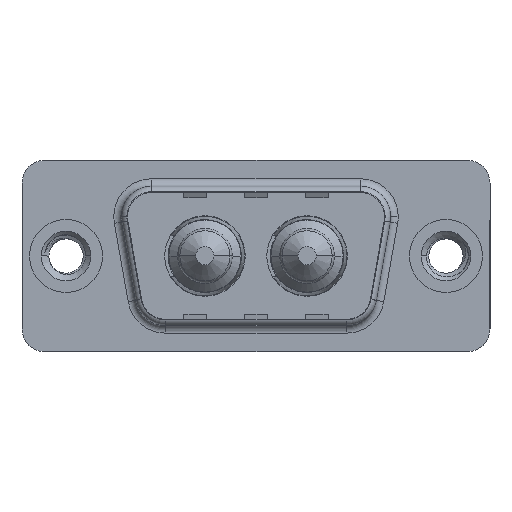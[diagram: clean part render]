
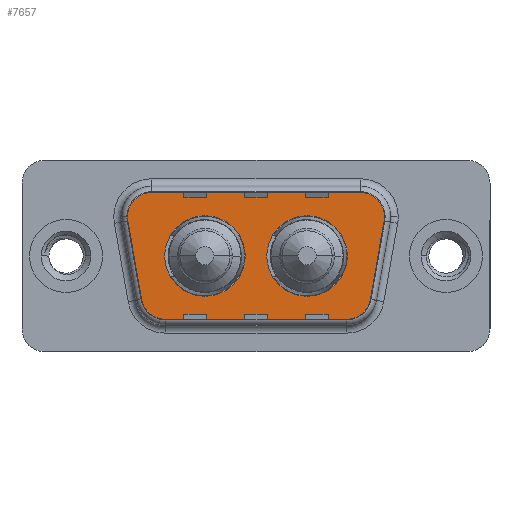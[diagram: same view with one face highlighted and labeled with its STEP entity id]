
A CAD part, top view. The second image highlights one B-rep face of the part: STEP entity #7657.
In plain terms, the highlighted planar face has unit normal (0, 0, 1).
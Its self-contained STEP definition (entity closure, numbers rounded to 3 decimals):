
#58 = VERTEX_POINT ( 'NONE', #12381 ) ;
#172 = AXIS2_PLACEMENT_3D ( 'NONE', #14242, #7520, #889 ) ;
#218 = VERTEX_POINT ( 'NONE', #12409 ) ;
#285 = FACE_OUTER_BOUND ( 'NONE', #12929, .T. ) ;
#431 = LINE ( 'NONE', #13626, #8936 ) ;
#558 = AXIS2_PLACEMENT_3D ( 'NONE', #10733, #6304, #14120 ) ;
#665 = ORIENTED_EDGE ( 'NONE', *, *, #1192, .T. ) ;
#889 = DIRECTION ( 'NONE',  ( -1., 0., 0. ) ) ;
#1007 = EDGE_CURVE ( 'NONE', #7636, #4635, #1743, .T. ) ;
#1170 = ORIENTED_EDGE ( 'NONE', *, *, #11515, .T. ) ;
#1192 = EDGE_CURVE ( 'NONE', #10052, #13337, #2941, .T. ) ;
#1240 = DIRECTION ( 'NONE',  ( -1., 0., 0. ) ) ;
#1664 = EDGE_LOOP ( 'NONE', ( #7968, #2176 ) ) ;
#1678 = ORIENTED_EDGE ( 'NONE', *, *, #3490, .F. ) ;
#1743 = LINE ( 'NONE', #14447, #13574 ) ;
#1864 = DIRECTION ( 'NONE',  ( 0., 0., 1. ) ) ;
#1905 = CIRCLE ( 'NONE', #172, 2. ) ;
#2075 = EDGE_CURVE ( 'NONE', #8472, #10052, #431, .T. ) ;
#2106 = EDGE_LOOP ( 'NONE', ( #1678, #3803 ) ) ;
#2176 = ORIENTED_EDGE ( 'NONE', *, *, #13136, .F. ) ;
#2181 = ORIENTED_EDGE ( 'NONE', *, *, #2075, .T. ) ;
#2243 = LINE ( 'NONE', #6777, #4479 ) ;
#2410 = AXIS2_PLACEMENT_3D ( 'NONE', #9677, #3035, #10810 ) ;
#2519 = CIRCLE ( 'NONE', #9203, 2. ) ;
#2628 = VERTEX_POINT ( 'NONE', #13806 ) ;
#2697 = CARTESIAN_POINT ( 'NONE',  ( 19.564, 4.9, 0. ) ) ;
#2818 = EDGE_CURVE ( 'NONE', #4635, #8472, #13822, .T. ) ;
#2941 = CIRCLE ( 'NONE', #11489, 2. ) ;
#3035 = DIRECTION ( 'NONE',  ( 0., 0., 1. ) ) ;
#3315 = VECTOR ( 'NONE', #6190, 1000. ) ;
#3490 = EDGE_CURVE ( 'NONE', #7587, #5668, #5252, .T. ) ;
#3670 = ORIENTED_EDGE ( 'NONE', *, *, #1007, .T. ) ;
#3803 = ORIENTED_EDGE ( 'NONE', *, *, #10053, .F. ) ;
#3835 = CARTESIAN_POINT ( 'NONE',  ( 11.79, 0., 0. ) ) ;
#4005 = CARTESIAN_POINT ( 'NONE',  ( 18.541, -2.9, 0. ) ) ;
#4009 = DIRECTION ( 'NONE',  ( 0., 0., 1. ) ) ;
#4071 = PLANE ( 'NONE',  #558 ) ;
#4243 = DIRECTION ( 'NONE',  ( 0., 0., 1. ) ) ;
#4479 = VECTOR ( 'NONE', #1240, 1000. ) ;
#4482 = CARTESIAN_POINT ( 'NONE',  ( 20.511, -3.247, 0. ) ) ;
#4635 = VERTEX_POINT ( 'NONE', #13031 ) ;
#4723 = DIRECTION ( 'NONE',  ( 0., 0., 1. ) ) ;
#5115 = DIRECTION ( 'NONE',  ( 1., 0., 0. ) ) ;
#5156 = VERTEX_POINT ( 'NONE', #2697 ) ;
#5252 = CIRCLE ( 'NONE', #2410, 2.65 ) ;
#5668 = VERTEX_POINT ( 'NONE', #14257 ) ;
#5886 = ORIENTED_EDGE ( 'NONE', *, *, #8289, .T. ) ;
#5939 = DIRECTION ( 'NONE',  ( 0., 0., 1. ) ) ;
#6101 = CARTESIAN_POINT ( 'NONE',  ( 18.51, 0., 0. ) ) ;
#6190 = DIRECTION ( 'NONE',  ( 0.174, -0.985, 0. ) ) ;
#6192 = EDGE_CURVE ( 'NONE', #58, #12251, #12219, .T. ) ;
#6210 = AXIS2_PLACEMENT_3D ( 'NONE', #8497, #1864, #9609 ) ;
#6238 = CARTESIAN_POINT ( 'NONE',  ( 5.436, 2.9, 0. ) ) ;
#6304 = DIRECTION ( 'NONE',  ( 0., 0., 1. ) ) ;
#6628 = DIRECTION ( 'NONE',  ( 1., 0., 0. ) ) ;
#6676 = EDGE_CURVE ( 'NONE', #14359, #2628, #8279, .T. ) ;
#6710 = AXIS2_PLACEMENT_3D ( 'NONE', #11413, #4723, #12542 ) ;
#6762 = AXIS2_PLACEMENT_3D ( 'NONE', #10913, #4243, #12054 ) ;
#6777 = CARTESIAN_POINT ( 'NONE',  ( 5.436, 4.9, 0. ) ) ;
#6885 = AXIS2_PLACEMENT_3D ( 'NONE', #12626, #5939, #13747 ) ;
#7348 = DIRECTION ( 'NONE',  ( 1., 0., 0. ) ) ;
#7361 = CARTESIAN_POINT ( 'NONE',  ( 6.459, -4.9, 0. ) ) ;
#7520 = DIRECTION ( 'NONE',  ( 0., 0., 1. ) ) ;
#7587 = VERTEX_POINT ( 'NONE', #6101 ) ;
#7618 = CARTESIAN_POINT ( 'NONE',  ( 21.564, 2.9, 0. ) ) ;
#7636 = VERTEX_POINT ( 'NONE', #7361 ) ;
#7657 = ADVANCED_FACE ( 'NONE', ( #14038, #8437, #285 ), #4071, .T. ) ;
#7886 = CIRCLE ( 'NONE', #6210, 2.65 ) ;
#7967 = CARTESIAN_POINT ( 'NONE',  ( 4.489, -3.247, 0. ) ) ;
#7968 = ORIENTED_EDGE ( 'NONE', *, *, #6676, .F. ) ;
#8046 = DIRECTION ( 'NONE',  ( 0.174, 0.985, 0. ) ) ;
#8279 = CIRCLE ( 'NONE', #6885, 2.65 ) ;
#8289 = EDGE_CURVE ( 'NONE', #218, #58, #2519, .T. ) ;
#8437 = FACE_BOUND ( 'NONE', #1664, .T. ) ;
#8472 = VERTEX_POINT ( 'NONE', #4482 ) ;
#8497 = CARTESIAN_POINT ( 'NONE',  ( 9.14, 0., 0. ) ) ;
#8530 = ORIENTED_EDGE ( 'NONE', *, *, #13390, .T. ) ;
#8936 = VECTOR ( 'NONE', #8046, 1000. ) ;
#9203 = AXIS2_PLACEMENT_3D ( 'NONE', #6238, #14055, #7348 ) ;
#9609 = DIRECTION ( 'NONE',  ( 1., 0., 0. ) ) ;
#9677 = CARTESIAN_POINT ( 'NONE',  ( 15.86, 0., 0. ) ) ;
#9725 = CARTESIAN_POINT ( 'NONE',  ( 21.534, 2.553, 0. ) ) ;
#9922 = ORIENTED_EDGE ( 'NONE', *, *, #2818, .T. ) ;
#10052 = VERTEX_POINT ( 'NONE', #9725 ) ;
#10053 = EDGE_CURVE ( 'NONE', #5668, #7587, #11940, .T. ) ;
#10623 = CARTESIAN_POINT ( 'NONE',  ( 3.466, 2.553, 0. ) ) ;
#10673 = CARTESIAN_POINT ( 'NONE',  ( 19.564, 2.9, 0. ) ) ;
#10688 = AXIS2_PLACEMENT_3D ( 'NONE', #4005, #11817, #5115 ) ;
#10733 = CARTESIAN_POINT ( 'NONE',  ( 18.541, -2.9, 0. ) ) ;
#10810 = DIRECTION ( 'NONE',  ( 1., 0., 0. ) ) ;
#10913 = CARTESIAN_POINT ( 'NONE',  ( 15.86, 0., 0. ) ) ;
#11062 = ORIENTED_EDGE ( 'NONE', *, *, #6192, .T. ) ;
#11383 = CIRCLE ( 'NONE', #6710, 2. ) ;
#11413 = CARTESIAN_POINT ( 'NONE',  ( 19.564, 2.9, 0. ) ) ;
#11489 = AXIS2_PLACEMENT_3D ( 'NONE', #10673, #4009, #11820 ) ;
#11515 = EDGE_CURVE ( 'NONE', #12251, #7636, #1905, .T. ) ;
#11817 = DIRECTION ( 'NONE',  ( 0., 0., 1. ) ) ;
#11820 = DIRECTION ( 'NONE',  ( -1., 0., 0. ) ) ;
#11940 = CIRCLE ( 'NONE', #6762, 2.65 ) ;
#12054 = DIRECTION ( 'NONE',  ( 1., 0., 0. ) ) ;
#12173 = EDGE_CURVE ( 'NONE', #5156, #218, #2243, .T. ) ;
#12219 = LINE ( 'NONE', #10623, #3315 ) ;
#12251 = VERTEX_POINT ( 'NONE', #7967 ) ;
#12381 = CARTESIAN_POINT ( 'NONE',  ( 3.466, 2.553, 0. ) ) ;
#12409 = CARTESIAN_POINT ( 'NONE',  ( 5.436, 4.9, 0. ) ) ;
#12504 = ORIENTED_EDGE ( 'NONE', *, *, #12173, .T. ) ;
#12542 = DIRECTION ( 'NONE',  ( -1., 0., 0. ) ) ;
#12626 = CARTESIAN_POINT ( 'NONE',  ( 9.14, 0., 0. ) ) ;
#12929 = EDGE_LOOP ( 'NONE', ( #9922, #2181, #665, #8530, #12504, #5886, #11062, #1170, #3670 ) ) ;
#13031 = CARTESIAN_POINT ( 'NONE',  ( 18.541, -4.9, 0. ) ) ;
#13136 = EDGE_CURVE ( 'NONE', #2628, #14359, #7886, .T. ) ;
#13337 = VERTEX_POINT ( 'NONE', #7618 ) ;
#13390 = EDGE_CURVE ( 'NONE', #13337, #5156, #11383, .T. ) ;
#13574 = VECTOR ( 'NONE', #6628, 1000. ) ;
#13626 = CARTESIAN_POINT ( 'NONE',  ( 21.534, 2.553, 0. ) ) ;
#13747 = DIRECTION ( 'NONE',  ( 1., 0., 0. ) ) ;
#13806 = CARTESIAN_POINT ( 'NONE',  ( 6.49, 0., 0. ) ) ;
#13822 = CIRCLE ( 'NONE', #10688, 2. ) ;
#14038 = FACE_BOUND ( 'NONE', #2106, .T. ) ;
#14055 = DIRECTION ( 'NONE',  ( 0., 0., 1. ) ) ;
#14120 = DIRECTION ( 'NONE',  ( 1., 0., 0. ) ) ;
#14242 = CARTESIAN_POINT ( 'NONE',  ( 6.459, -2.9, 0. ) ) ;
#14257 = CARTESIAN_POINT ( 'NONE',  ( 13.21, 0., 0. ) ) ;
#14359 = VERTEX_POINT ( 'NONE', #3835 ) ;
#14447 = CARTESIAN_POINT ( 'NONE',  ( 6.459, -4.9, 0. ) ) ;
